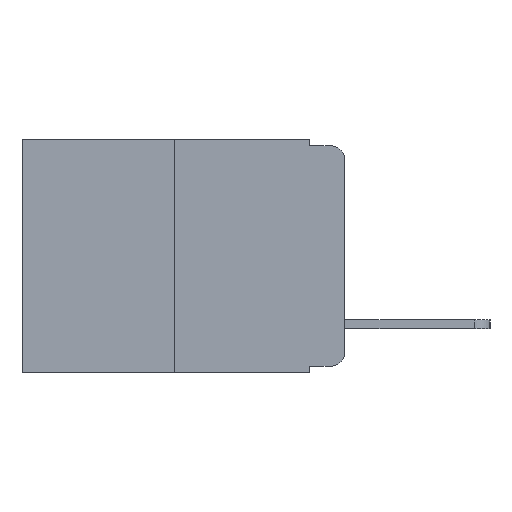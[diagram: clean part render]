
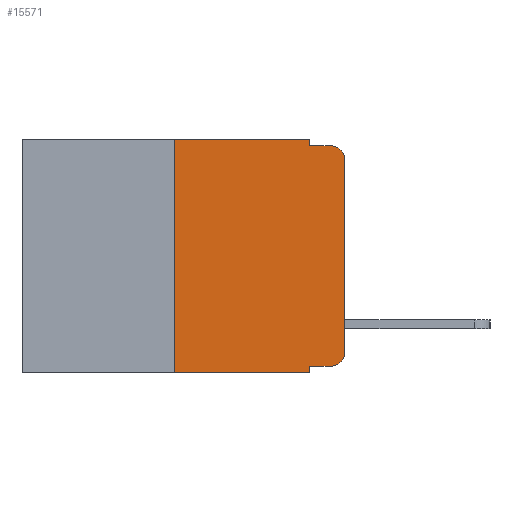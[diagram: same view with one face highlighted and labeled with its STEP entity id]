
A CAD part, left-side view. The second image highlights one B-rep face of the part: STEP entity #15571.
In plain terms, the highlighted planar face has unit normal (-1, 0, 0).
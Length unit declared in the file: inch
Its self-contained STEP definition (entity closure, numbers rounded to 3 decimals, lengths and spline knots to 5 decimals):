
#81 = VERTEX_POINT ( 'NONE', #4851 ) ;
#162 = CARTESIAN_POINT ( 'NONE',  ( 0., 0., -0.313 ) ) ;
#375 = VERTEX_POINT ( 'NONE', #4160 ) ;
#435 = ORIENTED_EDGE ( 'NONE', *, *, #17320, .F. ) ;
#876 = CARTESIAN_POINT ( 'NONE',  ( 0., 0.02, -0.03 ) ) ;
#1156 = DIRECTION ( 'NONE',  ( 0., 0., -1. ) ) ;
#1158 = FACE_OUTER_BOUND ( 'NONE', #13950, .T. ) ;
#1702 = VERTEX_POINT ( 'NONE', #19993 ) ;
#1985 = DIRECTION ( 'NONE',  ( 0., 0., -1. ) ) ;
#2033 = VERTEX_POINT ( 'NONE', #12081 ) ;
#2471 = VECTOR ( 'NONE', #14143, 39.37008 ) ;
#2495 = DIRECTION ( 'NONE',  ( 0., 0., -1. ) ) ;
#2614 = VECTOR ( 'NONE', #5035, 39.37008 ) ;
#3219 = VERTEX_POINT ( 'NONE', #14063 ) ;
#3339 = VERTEX_POINT ( 'NONE', #162 ) ;
#4160 = CARTESIAN_POINT ( 'NONE',  ( 0., 0.02, -0.333 ) ) ;
#4337 = VECTOR ( 'NONE', #15335, 39.37008 ) ;
#4851 = CARTESIAN_POINT ( 'NONE',  ( 0., 0.051, -0.333 ) ) ;
#5035 = DIRECTION ( 'NONE',  ( 0., -1., 0. ) ) ;
#5046 = AXIS2_PLACEMENT_3D ( 'NONE', #12116, #10567, #1156 ) ;
#5509 = CARTESIAN_POINT ( 'NONE',  ( 0., 0.02, -0.313 ) ) ;
#5556 = LINE ( 'NONE', #14197, #17361 ) ;
#5704 = CARTESIAN_POINT ( 'NONE',  ( 0., 0.051, 0. ) ) ;
#5843 = PLANE ( 'NONE',  #5046 ) ;
#6264 = VECTOR ( 'NONE', #15482, 39.37008 ) ;
#6537 = CARTESIAN_POINT ( 'NONE',  ( 0., 0.473, 0. ) ) ;
#6579 = LINE ( 'NONE', #18636, #2471 ) ;
#6966 = AXIS2_PLACEMENT_3D ( 'NONE', #5509, #16286, #6998 ) ;
#6998 = DIRECTION ( 'NONE',  ( 0., 0., -1. ) ) ;
#7427 = CARTESIAN_POINT ( 'NONE',  ( 0., 0.051, -0.01 ) ) ;
#8030 = VERTEX_POINT ( 'NONE', #5704 ) ;
#8427 = EDGE_CURVE ( 'NONE', #19806, #8030, #11466, .T. ) ;
#9227 = VERTEX_POINT ( 'NONE', #11208 ) ;
#10469 = LINE ( 'NONE', #12441, #6264 ) ;
#10567 = DIRECTION ( 'NONE',  ( 1., 0., 0. ) ) ;
#10775 = ORIENTED_EDGE ( 'NONE', *, *, #19057, .T. ) ;
#10925 = VECTOR ( 'NONE', #17685, 39.37008 ) ;
#11201 = DIRECTION ( 'NONE',  ( 0., 0., 1. ) ) ;
#11208 = CARTESIAN_POINT ( 'NONE',  ( 0., 0., -0.03 ) ) ;
#11320 = ORIENTED_EDGE ( 'NONE', *, *, #17119, .F. ) ;
#11466 = LINE ( 'NONE', #6537, #2614 ) ;
#11761 = CARTESIAN_POINT ( 'NONE',  ( 0., 0.051, -0.343 ) ) ;
#11828 = ORIENTED_EDGE ( 'NONE', *, *, #8427, .F. ) ;
#11923 = DIRECTION ( 'NONE',  ( -1., 0., 0. ) ) ;
#12081 = CARTESIAN_POINT ( 'NONE',  ( 0., 0.25, -0.343 ) ) ;
#12116 = CARTESIAN_POINT ( 'NONE',  ( 0., 0.473, 0. ) ) ;
#12404 = LINE ( 'NONE', #14338, #19838 ) ;
#12421 = CIRCLE ( 'NONE', #18437, 0.02 ) ;
#12441 = CARTESIAN_POINT ( 'NONE',  ( 0., 0.473, -0.343 ) ) ;
#13950 = EDGE_LOOP ( 'NONE', ( #10775, #19493, #16001, #11320, #11828, #17249, #19953, #435, #19297, #16044 ) ) ;
#13980 = CIRCLE ( 'NONE', #6966, 0.02 ) ;
#14002 = LINE ( 'NONE', #7427, #14482 ) ;
#14063 = CARTESIAN_POINT ( 'NONE',  ( 0., 0.02, -0.01 ) ) ;
#14143 = DIRECTION ( 'NONE',  ( 0., 0., 1. ) ) ;
#14197 = CARTESIAN_POINT ( 'NONE',  ( 0., 0.25, 0. ) ) ;
#14274 = VERTEX_POINT ( 'NONE', #11761 ) ;
#14338 = CARTESIAN_POINT ( 'NONE',  ( 0., 0.051, 0. ) ) ;
#14482 = VECTOR ( 'NONE', #18210, 39.37008 ) ;
#15335 = DIRECTION ( 'NONE',  ( 0., 0., -1. ) ) ;
#15482 = DIRECTION ( 'NONE',  ( 0., -1., 0. ) ) ;
#15571 = ADVANCED_FACE ( 'NONE', ( #1158 ), #5843, .F. ) ;
#15670 = CARTESIAN_POINT ( 'NONE',  ( 0., 0.25, 0. ) ) ;
#16001 = ORIENTED_EDGE ( 'NONE', *, *, #17067, .F. ) ;
#16044 = ORIENTED_EDGE ( 'NONE', *, *, #17408, .T. ) ;
#16130 = CARTESIAN_POINT ( 'NONE',  ( 0., 0.051, -0.333 ) ) ;
#16286 = DIRECTION ( 'NONE',  ( -1., 0., 0. ) ) ;
#16683 = EDGE_CURVE ( 'NONE', #2033, #14274, #10469, .T. ) ;
#16977 = EDGE_CURVE ( 'NONE', #9227, #3219, #12421, .T. ) ;
#17067 = EDGE_CURVE ( 'NONE', #1702, #3219, #14002, .T. ) ;
#17119 = EDGE_CURVE ( 'NONE', #8030, #1702, #17143, .T. ) ;
#17143 = LINE ( 'NONE', #18335, #4337 ) ;
#17249 = ORIENTED_EDGE ( 'NONE', *, *, #17269, .F. ) ;
#17269 = EDGE_CURVE ( 'NONE', #2033, #19806, #5556, .T. ) ;
#17320 = EDGE_CURVE ( 'NONE', #81, #14274, #12404, .T. ) ;
#17361 = VECTOR ( 'NONE', #11201, 39.37008 ) ;
#17379 = EDGE_CURVE ( 'NONE', #81, #375, #19386, .T. ) ;
#17408 = EDGE_CURVE ( 'NONE', #375, #3339, #13980, .T. ) ;
#17685 = DIRECTION ( 'NONE',  ( 0., -1., 0. ) ) ;
#18210 = DIRECTION ( 'NONE',  ( 0., -1., 0. ) ) ;
#18335 = CARTESIAN_POINT ( 'NONE',  ( 0., 0.051, 0. ) ) ;
#18437 = AXIS2_PLACEMENT_3D ( 'NONE', #876, #11923, #2495 ) ;
#18636 = CARTESIAN_POINT ( 'NONE',  ( 0., 0., 0. ) ) ;
#19057 = EDGE_CURVE ( 'NONE', #3339, #9227, #6579, .T. ) ;
#19297 = ORIENTED_EDGE ( 'NONE', *, *, #17379, .T. ) ;
#19386 = LINE ( 'NONE', #16130, #10925 ) ;
#19493 = ORIENTED_EDGE ( 'NONE', *, *, #16977, .T. ) ;
#19806 = VERTEX_POINT ( 'NONE', #15670 ) ;
#19838 = VECTOR ( 'NONE', #1985, 39.37008 ) ;
#19953 = ORIENTED_EDGE ( 'NONE', *, *, #16683, .T. ) ;
#19993 = CARTESIAN_POINT ( 'NONE',  ( 0., 0.051, -0.01 ) ) ;
